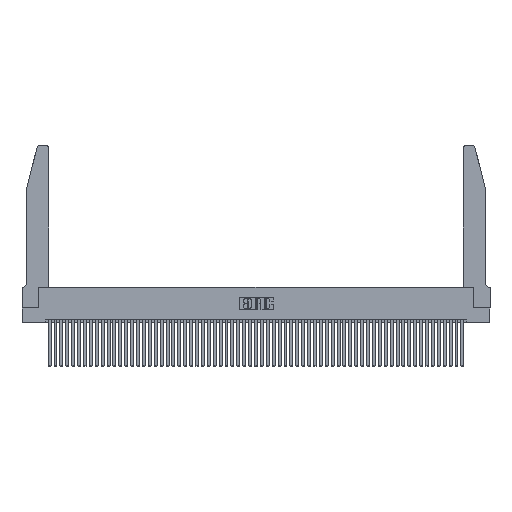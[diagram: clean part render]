
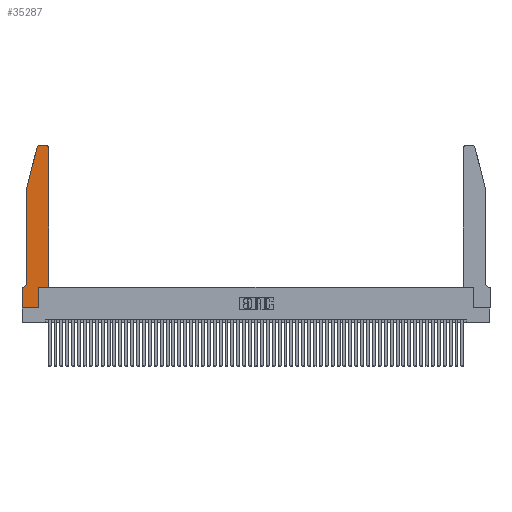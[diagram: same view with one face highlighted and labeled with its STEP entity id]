
A CAD part, top view. The second image highlights one B-rep face of the part: STEP entity #35287.
In plain terms, the highlighted planar face has unit normal (0, 0, 1).
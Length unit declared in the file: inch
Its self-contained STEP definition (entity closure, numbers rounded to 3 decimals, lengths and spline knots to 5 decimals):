
#649 = CARTESIAN_POINT ( 'NONE',  ( 0.284, 2.72, 0.37 ) ) ;
#1338 = CARTESIAN_POINT ( 'NONE',  ( 0.2865, 0.35, 0.37 ) ) ;
#2386 = VECTOR ( 'NONE', #49442, 39.37008 ) ;
#2547 = DIRECTION ( 'NONE',  ( 1., 0., 0. ) ) ;
#2908 = VERTEX_POINT ( 'NONE', #32272 ) ;
#3121 = ORIENTED_EDGE ( 'NONE', *, *, #31808, .T. ) ;
#3947 = VERTEX_POINT ( 'NONE', #35028 ) ;
#4111 = CIRCLE ( 'NONE', #29817, 0.03 ) ;
#4197 = VECTOR ( 'NONE', #52327, 39.37008 ) ;
#4344 = CARTESIAN_POINT ( 'NONE',  ( 0.0755, 0.42, 0.37 ) ) ;
#4844 = CIRCLE ( 'NONE', #14198, 0.03 ) ;
#5073 = DIRECTION ( 'NONE',  ( 1., 0., 0. ) ) ;
#5109 = CARTESIAN_POINT ( 'NONE',  ( 0.4505, 2.72, 0.37 ) ) ;
#6013 = CARTESIAN_POINT ( 'NONE',  ( 0.25487, 2.72718, 0.37 ) ) ;
#6511 = VERTEX_POINT ( 'NONE', #4344 ) ;
#6915 = LINE ( 'NONE', #21952, #4197 ) ;
#8325 = LINE ( 'NONE', #46266, #30159 ) ;
#9604 = CARTESIAN_POINT ( 'NONE',  ( 0.4505, 0.35, 0.37 ) ) ;
#10131 = DIRECTION ( 'NONE',  ( 0., 1., 0. ) ) ;
#10530 = ORIENTED_EDGE ( 'NONE', *, *, #37422, .T. ) ;
#10941 = CARTESIAN_POINT ( 'NONE',  ( 0., 0.35, 0.37 ) ) ;
#11294 = VECTOR ( 'NONE', #29869, 39.37008 ) ;
#12692 = ORIENTED_EDGE ( 'NONE', *, *, #19551, .T. ) ;
#13215 = VERTEX_POINT ( 'NONE', #26547 ) ;
#13273 = DIRECTION ( 'NONE',  ( 1., 0., 0. ) ) ;
#13608 = DIRECTION ( 'NONE',  ( -0.239, -0.971, 0. ) ) ;
#13830 = VERTEX_POINT ( 'NONE', #17390 ) ;
#14198 = AXIS2_PLACEMENT_3D ( 'NONE', #649, #31161, #5073 ) ;
#15540 = EDGE_CURVE ( 'NONE', #30263, #24513, #4111, .T. ) ;
#15887 = ORIENTED_EDGE ( 'NONE', *, *, #44284, .T. ) ;
#17390 = CARTESIAN_POINT ( 'NONE',  ( 0.0055, 0.35, 0.37 ) ) ;
#18005 = CARTESIAN_POINT ( 'NONE',  ( 0.0755, 2., 0.37 ) ) ;
#18762 = EDGE_CURVE ( 'NONE', #49242, #18956, #4844, .T. ) ;
#18832 = CARTESIAN_POINT ( 'NONE',  ( 0.284, 2.75, 0.37 ) ) ;
#18956 = VERTEX_POINT ( 'NONE', #6013 ) ;
#18985 = CARTESIAN_POINT ( 'NONE',  ( 0., 0., 0.37 ) ) ;
#19374 = DIRECTION ( 'NONE',  ( -1., 0., 0. ) ) ;
#19402 = ORIENTED_EDGE ( 'NONE', *, *, #18762, .T. ) ;
#19551 = EDGE_CURVE ( 'NONE', #2908, #3947, #20461, .T. ) ;
#19681 = CARTESIAN_POINT ( 'NONE',  ( 0.0055, 0.42, 0.37 ) ) ;
#19931 = PLANE ( 'NONE',  #31375 ) ;
#20461 = LINE ( 'NONE', #1338, #42189 ) ;
#21514 = LINE ( 'NONE', #32488, #33065 ) ;
#21569 = LINE ( 'NONE', #55892, #11294 ) ;
#21823 = EDGE_CURVE ( 'NONE', #54636, #6511, #21569, .T. ) ;
#21949 = EDGE_LOOP ( 'NONE', ( #48657, #19402, #15887, #47217, #41059, #10530, #3121, #53504, #12692, #35848, #39144, #44614 ) ) ;
#21952 = CARTESIAN_POINT ( 'NONE',  ( 0.0755, 0.35, 0.37 ) ) ;
#22257 = EDGE_CURVE ( 'NONE', #24513, #49242, #21514, .T. ) ;
#24072 = DIRECTION ( 'NONE',  ( -1., 0., 0. ) ) ;
#24513 = VERTEX_POINT ( 'NONE', #38845 ) ;
#25479 = CARTESIAN_POINT ( 'NONE',  ( 0.4205, 2.72, 0.37 ) ) ;
#26547 = CARTESIAN_POINT ( 'NONE',  ( 0., 0.35, 0.37 ) ) ;
#28320 = LINE ( 'NONE', #45060, #2386 ) ;
#28658 = DIRECTION ( 'NONE',  ( 0., 0., 1. ) ) ;
#28773 = DIRECTION ( 'NONE',  ( 0., -1., 0. ) ) ;
#29070 = VERTEX_POINT ( 'NONE', #43720 ) ;
#29817 = AXIS2_PLACEMENT_3D ( 'NONE', #25479, #55857, #29836 ) ;
#29836 = DIRECTION ( 'NONE',  ( 1., 0., 0. ) ) ;
#29869 = DIRECTION ( 'NONE',  ( 0., -1., 0. ) ) ;
#30159 = VECTOR ( 'NONE', #28773, 39.37008 ) ;
#30263 = VERTEX_POINT ( 'NONE', #5109 ) ;
#30721 = EDGE_CURVE ( 'NONE', #36272, #2908, #51362, .T. ) ;
#31161 = DIRECTION ( 'NONE',  ( 0., 0., 1. ) ) ;
#31375 = AXIS2_PLACEMENT_3D ( 'NONE', #10941, #28658, #2547 ) ;
#31808 = EDGE_CURVE ( 'NONE', #13215, #36272, #8325, .T. ) ;
#32272 = CARTESIAN_POINT ( 'NONE',  ( 0.2865, 0., 0.37 ) ) ;
#32488 = CARTESIAN_POINT ( 'NONE',  ( 0.2605, 2.75, 0.37 ) ) ;
#33065 = VECTOR ( 'NONE', #19374, 39.37008 ) ;
#34198 = LINE ( 'NONE', #9604, #55923 ) ;
#35028 = CARTESIAN_POINT ( 'NONE',  ( 0.2865, 0.35, 0.37 ) ) ;
#35287 = ADVANCED_FACE ( 'NONE', ( #51598 ), #19931, .T. ) ;
#35763 = VECTOR ( 'NONE', #13608, 39.37008 ) ;
#35848 = ORIENTED_EDGE ( 'NONE', *, *, #46206, .T. ) ;
#36272 = VERTEX_POINT ( 'NONE', #18985 ) ;
#37422 = EDGE_CURVE ( 'NONE', #13830, #13215, #6915, .T. ) ;
#38845 = CARTESIAN_POINT ( 'NONE',  ( 0.4205, 2.75, 0.37 ) ) ;
#38956 = CIRCLE ( 'NONE', #47962, 0.07 ) ;
#39144 = ORIENTED_EDGE ( 'NONE', *, *, #41767, .T. ) ;
#39780 = VECTOR ( 'NONE', #13273, 39.37008 ) ;
#41059 = ORIENTED_EDGE ( 'NONE', *, *, #52730, .T. ) ;
#41767 = EDGE_CURVE ( 'NONE', #29070, #30263, #28320, .T. ) ;
#42189 = VECTOR ( 'NONE', #10131, 39.37008 ) ;
#43540 = CARTESIAN_POINT ( 'NONE',  ( 0., 0., 0.37 ) ) ;
#43720 = CARTESIAN_POINT ( 'NONE',  ( 0.4505, 0.35, 0.37 ) ) ;
#44257 = DIRECTION ( 'NONE',  ( 1., 0., 0. ) ) ;
#44284 = EDGE_CURVE ( 'NONE', #18956, #54636, #47333, .T. ) ;
#44614 = ORIENTED_EDGE ( 'NONE', *, *, #15540, .T. ) ;
#45060 = CARTESIAN_POINT ( 'NONE',  ( 0.4505, 0.35, 0.37 ) ) ;
#46206 = EDGE_CURVE ( 'NONE', #3947, #29070, #34198, .T. ) ;
#46266 = CARTESIAN_POINT ( 'NONE',  ( 0., 0., 0.37 ) ) ;
#47217 = ORIENTED_EDGE ( 'NONE', *, *, #21823, .T. ) ;
#47333 = LINE ( 'NONE', #18005, #35763 ) ;
#47962 = AXIS2_PLACEMENT_3D ( 'NONE', #19681, #50092, #24072 ) ;
#48657 = ORIENTED_EDGE ( 'NONE', *, *, #22257, .T. ) ;
#49242 = VERTEX_POINT ( 'NONE', #18832 ) ;
#49442 = DIRECTION ( 'NONE',  ( 0., 1., 0. ) ) ;
#49796 = CARTESIAN_POINT ( 'NONE',  ( 0.0755, 2., 0.37 ) ) ;
#50092 = DIRECTION ( 'NONE',  ( 0., 0., -1. ) ) ;
#51362 = LINE ( 'NONE', #43540, #39780 ) ;
#51598 = FACE_OUTER_BOUND ( 'NONE', #21949, .T. ) ;
#52327 = DIRECTION ( 'NONE',  ( -1., 0., 0. ) ) ;
#52730 = EDGE_CURVE ( 'NONE', #6511, #13830, #38956, .T. ) ;
#53504 = ORIENTED_EDGE ( 'NONE', *, *, #30721, .T. ) ;
#54636 = VERTEX_POINT ( 'NONE', #49796 ) ;
#55857 = DIRECTION ( 'NONE',  ( 0., 0., 1. ) ) ;
#55892 = CARTESIAN_POINT ( 'NONE',  ( 0.0755, 2., 0.37 ) ) ;
#55923 = VECTOR ( 'NONE', #44257, 39.37008 ) ;
